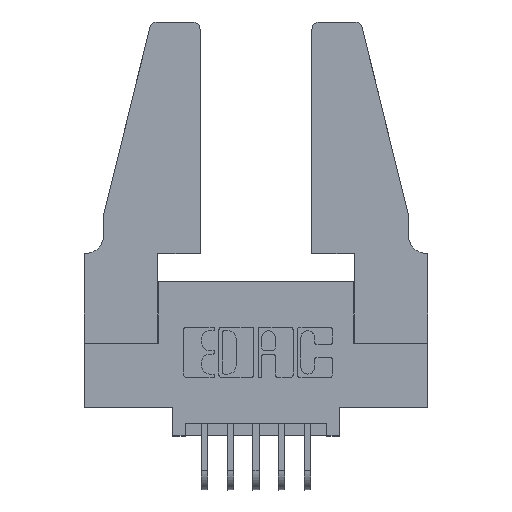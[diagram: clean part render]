
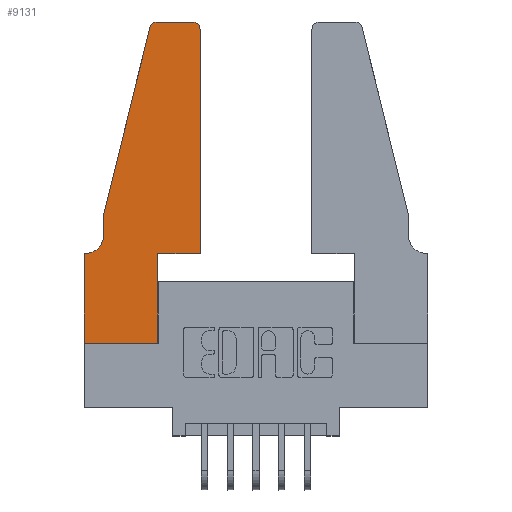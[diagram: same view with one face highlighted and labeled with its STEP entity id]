
A CAD part, top view. The second image highlights one B-rep face of the part: STEP entity #9131.
In plain terms, the highlighted planar face has unit normal (0, 0, 1).
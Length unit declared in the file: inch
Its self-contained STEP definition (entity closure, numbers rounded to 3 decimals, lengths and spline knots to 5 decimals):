
#151 = VERTEX_POINT ( 'NONE', #5807 ) ;
#166 = CARTESIAN_POINT ( 'NONE',  ( 0., 0.35, 0.37 ) ) ;
#283 = EDGE_CURVE ( 'NONE', #4624, #1895, #3420, .T. ) ;
#296 = LINE ( 'NONE', #6288, #4627 ) ;
#395 = LINE ( 'NONE', #879, #6600 ) ;
#443 = CARTESIAN_POINT ( 'NONE',  ( 0.2865, 0.35, 0.37 ) ) ;
#506 = VECTOR ( 'NONE', #5989, 39.37008 ) ;
#662 = ORIENTED_EDGE ( 'NONE', *, *, #11979, .T. ) ;
#772 = FACE_OUTER_BOUND ( 'NONE', #11851, .T. ) ;
#879 = CARTESIAN_POINT ( 'NONE',  ( 0., 0., 0.37 ) ) ;
#990 = ORIENTED_EDGE ( 'NONE', *, *, #12715, .T. ) ;
#1382 = VECTOR ( 'NONE', #12177, 39.37008 ) ;
#1473 = VERTEX_POINT ( 'NONE', #9628 ) ;
#1895 = VERTEX_POINT ( 'NONE', #10484 ) ;
#2059 = LINE ( 'NONE', #4959, #12478 ) ;
#2238 = VECTOR ( 'NONE', #11265, 39.37008 ) ;
#2291 = AXIS2_PLACEMENT_3D ( 'NONE', #10405, #3837, #6224 ) ;
#2361 = DIRECTION ( 'NONE',  ( 1., 0., 0. ) ) ;
#2364 = LINE ( 'NONE', #9963, #506 ) ;
#2450 = VERTEX_POINT ( 'NONE', #8411 ) ;
#2513 = DIRECTION ( 'NONE',  ( 1., 0., 0. ) ) ;
#2563 = ORIENTED_EDGE ( 'NONE', *, *, #8052, .T. ) ;
#2679 = VERTEX_POINT ( 'NONE', #3830 ) ;
#3120 = VECTOR ( 'NONE', #7983, 39.37008 ) ;
#3390 = LINE ( 'NONE', #5262, #1382 ) ;
#3420 = LINE ( 'NONE', #10956, #3120 ) ;
#3472 = PLANE ( 'NONE',  #2291 ) ;
#3662 = CARTESIAN_POINT ( 'NONE',  ( 0.0755, 0.5, 0.37 ) ) ;
#3748 = CARTESIAN_POINT ( 'NONE',  ( 0.4505, 0.35, 0.37 ) ) ;
#3830 = CARTESIAN_POINT ( 'NONE',  ( 0.0055, 0.35, 0.37 ) ) ;
#3837 = DIRECTION ( 'NONE',  ( 0., 0., 1. ) ) ;
#4027 = EDGE_CURVE ( 'NONE', #9029, #10264, #6929, .T. ) ;
#4157 = CARTESIAN_POINT ( 'NONE',  ( 0.0055, 0.42, 0.37 ) ) ;
#4393 = VERTEX_POINT ( 'NONE', #166 ) ;
#4426 = ORIENTED_EDGE ( 'NONE', *, *, #6196, .T. ) ;
#4624 = VERTEX_POINT ( 'NONE', #3748 ) ;
#4627 = VECTOR ( 'NONE', #7330, 39.37008 ) ;
#4959 = CARTESIAN_POINT ( 'NONE',  ( 0.0755, 0.5, 0.37 ) ) ;
#5262 = CARTESIAN_POINT ( 'NONE',  ( 0.0755, 0.35, 0.37 ) ) ;
#5613 = ORIENTED_EDGE ( 'NONE', *, *, #9910, .T. ) ;
#5807 = CARTESIAN_POINT ( 'NONE',  ( 0.0755, 0.42, 0.37 ) ) ;
#5975 = ORIENTED_EDGE ( 'NONE', *, *, #8606, .T. ) ;
#5987 = DIRECTION ( 'NONE',  ( -0.239, -0.971, 0. ) ) ;
#5989 = DIRECTION ( 'NONE',  ( 0., -1., 0. ) ) ;
#6152 = DIRECTION ( 'NONE',  ( 0., 0., -1. ) ) ;
#6196 = EDGE_CURVE ( 'NONE', #1473, #9029, #395, .T. ) ;
#6224 = DIRECTION ( 'NONE',  ( 1., 0., 0. ) ) ;
#6288 = CARTESIAN_POINT ( 'NONE',  ( 0.2605, 1.25, 0.37 ) ) ;
#6394 = VECTOR ( 'NONE', #7761, 39.37008 ) ;
#6549 = ORIENTED_EDGE ( 'NONE', *, *, #9743, .T. ) ;
#6600 = VECTOR ( 'NONE', #10815, 39.37008 ) ;
#6873 = VERTEX_POINT ( 'NONE', #12872 ) ;
#6929 = LINE ( 'NONE', #443, #2238 ) ;
#7176 = AXIS2_PLACEMENT_3D ( 'NONE', #10344, #8349, #2513 ) ;
#7219 = DIRECTION ( 'NONE',  ( 0., 0., 1. ) ) ;
#7330 = DIRECTION ( 'NONE',  ( -1., 0., 0. ) ) ;
#7357 = EDGE_CURVE ( 'NONE', #11275, #10473, #2059, .T. ) ;
#7631 = CARTESIAN_POINT ( 'NONE',  ( 0.0755, 0.5, 0.37 ) ) ;
#7632 = LINE ( 'NONE', #9900, #8891 ) ;
#7761 = DIRECTION ( 'NONE',  ( 0., -1., 0. ) ) ;
#7815 = DIRECTION ( 'NONE',  ( 1., 0., 0. ) ) ;
#7824 = ORIENTED_EDGE ( 'NONE', *, *, #4027, .T. ) ;
#7929 = ORIENTED_EDGE ( 'NONE', *, *, #11788, .T. ) ;
#7983 = DIRECTION ( 'NONE',  ( 0., 1., 0. ) ) ;
#8052 = EDGE_CURVE ( 'NONE', #1895, #6873, #9471, .T. ) ;
#8349 = DIRECTION ( 'NONE',  ( 0., 0., 1. ) ) ;
#8411 = CARTESIAN_POINT ( 'NONE',  ( 0.284, 1.25, 0.37 ) ) ;
#8439 = AXIS2_PLACEMENT_3D ( 'NONE', #4157, #6152, #10003 ) ;
#8606 = EDGE_CURVE ( 'NONE', #151, #2679, #12292, .T. ) ;
#8891 = VECTOR ( 'NONE', #7815, 39.37008 ) ;
#9029 = VERTEX_POINT ( 'NONE', #10897 ) ;
#9131 = ADVANCED_FACE ( 'NONE', ( #772 ), #3472, .T. ) ;
#9471 = CIRCLE ( 'NONE', #11523, 0.03 ) ;
#9628 = CARTESIAN_POINT ( 'NONE',  ( 0., 0., 0.37 ) ) ;
#9629 = ORIENTED_EDGE ( 'NONE', *, *, #12307, .T. ) ;
#9743 = EDGE_CURVE ( 'NONE', #6873, #2450, #296, .T. ) ;
#9820 = CIRCLE ( 'NONE', #7176, 0.03 ) ;
#9900 = CARTESIAN_POINT ( 'NONE',  ( 0.4505, 0.35, 0.37 ) ) ;
#9910 = EDGE_CURVE ( 'NONE', #2679, #4393, #3390, .T. ) ;
#9963 = CARTESIAN_POINT ( 'NONE',  ( 0., 0., 0.37 ) ) ;
#10003 = DIRECTION ( 'NONE',  ( -1., 0., 0. ) ) ;
#10264 = VERTEX_POINT ( 'NONE', #12232 ) ;
#10268 = LINE ( 'NONE', #7631, #6394 ) ;
#10344 = CARTESIAN_POINT ( 'NONE',  ( 0.284, 1.22, 0.37 ) ) ;
#10405 = CARTESIAN_POINT ( 'NONE',  ( 0., 0.35, 0.37 ) ) ;
#10473 = VERTEX_POINT ( 'NONE', #3662 ) ;
#10484 = CARTESIAN_POINT ( 'NONE',  ( 0.4505, 1.22, 0.37 ) ) ;
#10815 = DIRECTION ( 'NONE',  ( 1., 0., 0. ) ) ;
#10897 = CARTESIAN_POINT ( 'NONE',  ( 0.2865, 0., 0.37 ) ) ;
#10956 = CARTESIAN_POINT ( 'NONE',  ( 0.4505, 0.35, 0.37 ) ) ;
#11170 = CARTESIAN_POINT ( 'NONE',  ( 0.25487, 1.22718, 0.37 ) ) ;
#11217 = ORIENTED_EDGE ( 'NONE', *, *, #7357, .T. ) ;
#11242 = CARTESIAN_POINT ( 'NONE',  ( 0.4205, 1.22, 0.37 ) ) ;
#11265 = DIRECTION ( 'NONE',  ( 0., 1., 0. ) ) ;
#11275 = VERTEX_POINT ( 'NONE', #11170 ) ;
#11523 = AXIS2_PLACEMENT_3D ( 'NONE', #11242, #7219, #2361 ) ;
#11681 = ORIENTED_EDGE ( 'NONE', *, *, #283, .T. ) ;
#11788 = EDGE_CURVE ( 'NONE', #4393, #1473, #2364, .T. ) ;
#11851 = EDGE_LOOP ( 'NONE', ( #6549, #662, #11217, #990, #5975, #5613, #7929, #4426, #7824, #9629, #11681, #2563 ) ) ;
#11979 = EDGE_CURVE ( 'NONE', #2450, #11275, #9820, .T. ) ;
#12177 = DIRECTION ( 'NONE',  ( -1., 0., 0. ) ) ;
#12232 = CARTESIAN_POINT ( 'NONE',  ( 0.2865, 0.35, 0.37 ) ) ;
#12292 = CIRCLE ( 'NONE', #8439, 0.07 ) ;
#12307 = EDGE_CURVE ( 'NONE', #10264, #4624, #7632, .T. ) ;
#12478 = VECTOR ( 'NONE', #5987, 39.37008 ) ;
#12715 = EDGE_CURVE ( 'NONE', #10473, #151, #10268, .T. ) ;
#12872 = CARTESIAN_POINT ( 'NONE',  ( 0.4205, 1.25, 0.37 ) ) ;
